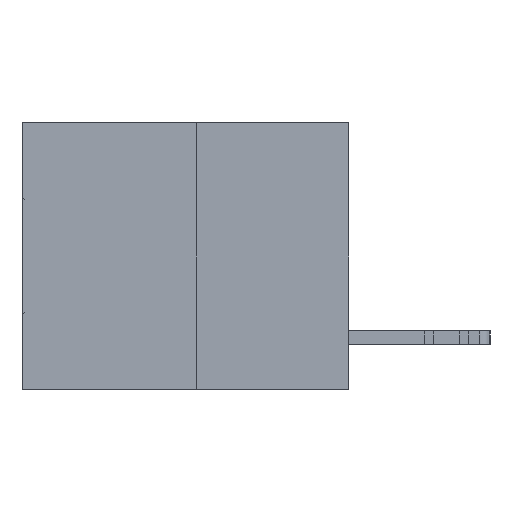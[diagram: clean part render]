
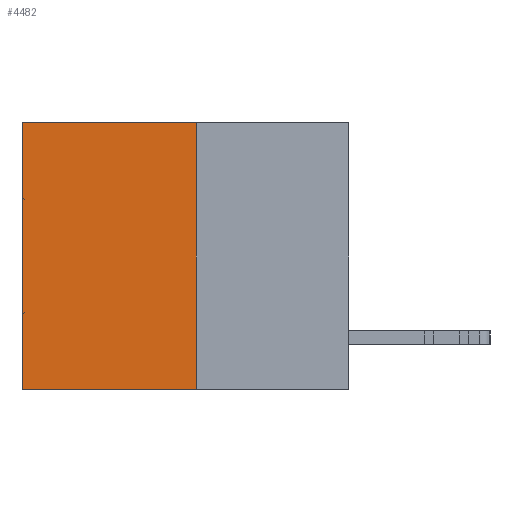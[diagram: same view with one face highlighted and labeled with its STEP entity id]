
A CAD part, left-side view. The second image highlights one B-rep face of the part: STEP entity #4482.
In plain terms, the highlighted planar face has unit normal (-1, 0, 0).
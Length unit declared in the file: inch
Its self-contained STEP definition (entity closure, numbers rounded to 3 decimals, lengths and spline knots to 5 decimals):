
#342 = DIRECTION ( 'NONE',  ( 1., 0., 0. ) ) ;
#1570 = CARTESIAN_POINT ( 'NONE',  ( 0.3165, 0.28, -0.49 ) ) ;
#2828 = VERTEX_POINT ( 'NONE', #8658 ) ;
#3300 = ORIENTED_EDGE ( 'NONE', *, *, #30798, .T. ) ;
#3337 = VERTEX_POINT ( 'NONE', #4991 ) ;
#4482 = ADVANCED_FACE ( 'NONE', ( #28409 ), #10025, .F. ) ;
#4991 = CARTESIAN_POINT ( 'NONE',  ( 0.3165, 0.6, -0.49 ) ) ;
#5265 = LINE ( 'NONE', #7564, #23513 ) ;
#5708 = LINE ( 'NONE', #24962, #6457 ) ;
#6457 = VECTOR ( 'NONE', #27770, 39.37008 ) ;
#6718 = ORIENTED_EDGE ( 'NONE', *, *, #7289, .F. ) ;
#7289 = EDGE_CURVE ( 'NONE', #2828, #3337, #16334, .T. ) ;
#7564 = CARTESIAN_POINT ( 'NONE',  ( 0.3165, 0.6, -0.49 ) ) ;
#7975 = VERTEX_POINT ( 'NONE', #21101 ) ;
#8658 = CARTESIAN_POINT ( 'NONE',  ( 0.3165, 0.28, -0.49 ) ) ;
#8764 = ORIENTED_EDGE ( 'NONE', *, *, #14779, .T. ) ;
#10025 = PLANE ( 'NONE',  #11107 ) ;
#11107 = AXIS2_PLACEMENT_3D ( 'NONE', #12395, #342, #21706 ) ;
#12395 = CARTESIAN_POINT ( 'NONE',  ( 0.3165, 0.28, -0.49 ) ) ;
#13316 = DIRECTION ( 'NONE',  ( 0., 1., 0. ) ) ;
#13632 = CARTESIAN_POINT ( 'NONE',  ( 0.3165, 0.28, 0. ) ) ;
#14779 = EDGE_CURVE ( 'NONE', #7975, #23726, #20947, .T. ) ;
#16307 = DIRECTION ( 'NONE',  ( 0., 1., 0. ) ) ;
#16334 = LINE ( 'NONE', #1570, #25383 ) ;
#18426 = EDGE_CURVE ( 'NONE', #7975, #2828, #5708, .T. ) ;
#19250 = ORIENTED_EDGE ( 'NONE', *, *, #18426, .F. ) ;
#19818 = VECTOR ( 'NONE', #13316, 39.37008 ) ;
#20611 = EDGE_LOOP ( 'NONE', ( #3300, #6718, #19250, #8764 ) ) ;
#20947 = LINE ( 'NONE', #13632, #19818 ) ;
#21101 = CARTESIAN_POINT ( 'NONE',  ( 0.3165, 0.28, 0. ) ) ;
#21706 = DIRECTION ( 'NONE',  ( 0., 0., -1. ) ) ;
#22770 = CARTESIAN_POINT ( 'NONE',  ( 0.3165, 0.6, 0. ) ) ;
#23513 = VECTOR ( 'NONE', #24573, 39.37008 ) ;
#23726 = VERTEX_POINT ( 'NONE', #22770 ) ;
#24573 = DIRECTION ( 'NONE',  ( 0., 0., -1. ) ) ;
#24962 = CARTESIAN_POINT ( 'NONE',  ( 0.3165, 0.28, -0.49 ) ) ;
#25383 = VECTOR ( 'NONE', #16307, 39.37008 ) ;
#27770 = DIRECTION ( 'NONE',  ( 0., 0., -1. ) ) ;
#28409 = FACE_OUTER_BOUND ( 'NONE', #20611, .T. ) ;
#30798 = EDGE_CURVE ( 'NONE', #23726, #3337, #5265, .T. ) ;
